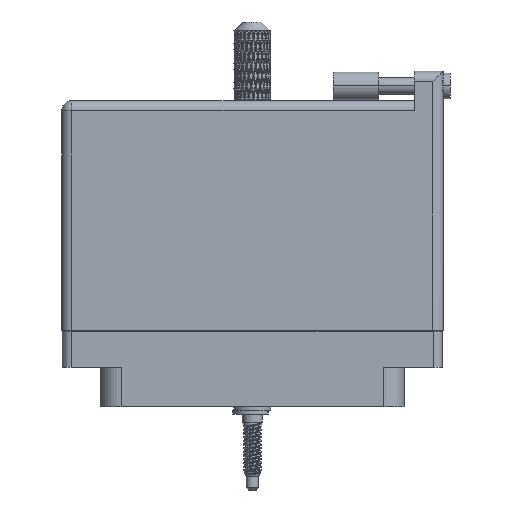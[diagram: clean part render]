
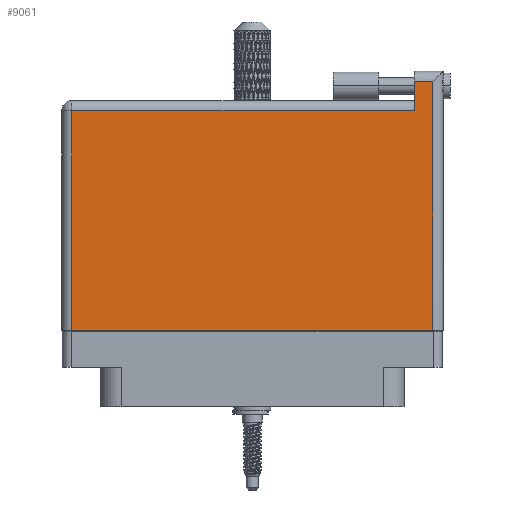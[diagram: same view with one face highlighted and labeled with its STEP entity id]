
A CAD part, front view. The second image highlights one B-rep face of the part: STEP entity #9061.
In plain terms, the highlighted face is planar.
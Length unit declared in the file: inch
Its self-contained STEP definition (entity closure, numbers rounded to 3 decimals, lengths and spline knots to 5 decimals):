
#241 = DIRECTION ( 'NONE',  ( 0., 1., 0. ) ) ;
#4045 = CARTESIAN_POINT ( 'NONE',  ( 1.103, 1.596, 0.4495 ) ) ;
#4358 = VECTOR ( 'NONE', #71319, 39.37008 ) ;
#5617 = CARTESIAN_POINT ( 'NONE',  ( -1.23, -0.1, 0.4495 ) ) ;
#9061 = ADVANCED_FACE ( 'NONE', ( #14877 ), #100077, .F. ) ;
#9693 = ORIENTED_EDGE ( 'NONE', *, *, #110817, .T. ) ;
#12129 = EDGE_CURVE ( 'NONE', #85613, #95879, #25515, .T. ) ;
#14457 = AXIS2_PLACEMENT_3D ( 'NONE', #73608, #91419, #43045 ) ;
#14877 = FACE_OUTER_BOUND ( 'NONE', #95037, .T. ) ;
#16891 = VECTOR ( 'NONE', #107130, 39.37008 ) ;
#17241 = VERTEX_POINT ( 'NONE', #61958 ) ;
#19607 = EDGE_CURVE ( 'NONE', #89083, #38922, #87754, .T. ) ;
#19881 = CARTESIAN_POINT ( 'NONE',  ( -1.23, 1.396, 0.4495 ) ) ;
#20017 = CARTESIAN_POINT ( 'NONE',  ( 1.23, -0.1, 0.4495 ) ) ;
#22620 = VECTOR ( 'NONE', #49293, 39.37008 ) ;
#22822 = LINE ( 'NONE', #43887, #4358 ) ;
#23565 = VERTEX_POINT ( 'NONE', #19881 ) ;
#25515 = LINE ( 'NONE', #94495, #22620 ) ;
#32418 = EDGE_CURVE ( 'NONE', #95879, #89083, #117446, .T. ) ;
#35623 = CARTESIAN_POINT ( 'NONE',  ( 1.23, 1.666, 0.4495 ) ) ;
#38922 = VERTEX_POINT ( 'NONE', #4045 ) ;
#41634 = DIRECTION ( 'NONE',  ( 0., -1., 0. ) ) ;
#43045 = DIRECTION ( 'NONE',  ( -1., 0., 0. ) ) ;
#43887 = CARTESIAN_POINT ( 'NONE',  ( -1.3, 1.396, 0.4495 ) ) ;
#45100 = VECTOR ( 'NONE', #241, 39.37008 ) ;
#49293 = DIRECTION ( 'NONE',  ( 1., 0., 0. ) ) ;
#58552 = CARTESIAN_POINT ( 'NONE',  ( -1.23, -0.1, 0.4495 ) ) ;
#59742 = VECTOR ( 'NONE', #86819, 39.37008 ) ;
#61958 = CARTESIAN_POINT ( 'NONE',  ( 1.103, 1.396, 0.4495 ) ) ;
#71319 = DIRECTION ( 'NONE',  ( -1., 0., 0. ) ) ;
#73608 = CARTESIAN_POINT ( 'NONE',  ( -1.3, 1.466, 0.4495 ) ) ;
#82462 = LINE ( 'NONE', #5617, #59742 ) ;
#85613 = VERTEX_POINT ( 'NONE', #58552 ) ;
#86819 = DIRECTION ( 'NONE',  ( 0., -1., 0. ) ) ;
#87754 = LINE ( 'NONE', #106746, #16891 ) ;
#89083 = VERTEX_POINT ( 'NONE', #93434 ) ;
#91419 = DIRECTION ( 'NONE',  ( 0., 0., -1. ) ) ;
#93434 = CARTESIAN_POINT ( 'NONE',  ( 1.23, 1.596, 0.4495 ) ) ;
#94495 = CARTESIAN_POINT ( 'NONE',  ( -1.3, -0.1, 0.4495 ) ) ;
#95037 = EDGE_LOOP ( 'NONE', ( #106089, #107167, #96301, #96518, #9693, #112054 ) ) ;
#95879 = VERTEX_POINT ( 'NONE', #20017 ) ;
#96301 = ORIENTED_EDGE ( 'NONE', *, *, #19607, .T. ) ;
#96518 = ORIENTED_EDGE ( 'NONE', *, *, #101482, .T. ) ;
#100077 = PLANE ( 'NONE',  #14457 ) ;
#101482 = EDGE_CURVE ( 'NONE', #38922, #17241, #116083, .T. ) ;
#106089 = ORIENTED_EDGE ( 'NONE', *, *, #12129, .T. ) ;
#106746 = CARTESIAN_POINT ( 'NONE',  ( -1.3, 1.596, 0.4495 ) ) ;
#107130 = DIRECTION ( 'NONE',  ( -1., 0., 0. ) ) ;
#107167 = ORIENTED_EDGE ( 'NONE', *, *, #32418, .T. ) ;
#110273 = EDGE_CURVE ( 'NONE', #23565, #85613, #82462, .T. ) ;
#110339 = VECTOR ( 'NONE', #41634, 39.37008 ) ;
#110817 = EDGE_CURVE ( 'NONE', #17241, #23565, #22822, .T. ) ;
#111062 = CARTESIAN_POINT ( 'NONE',  ( 1.103, 1.666, 0.4495 ) ) ;
#112054 = ORIENTED_EDGE ( 'NONE', *, *, #110273, .T. ) ;
#116083 = LINE ( 'NONE', #111062, #110339 ) ;
#117446 = LINE ( 'NONE', #35623, #45100 ) ;
